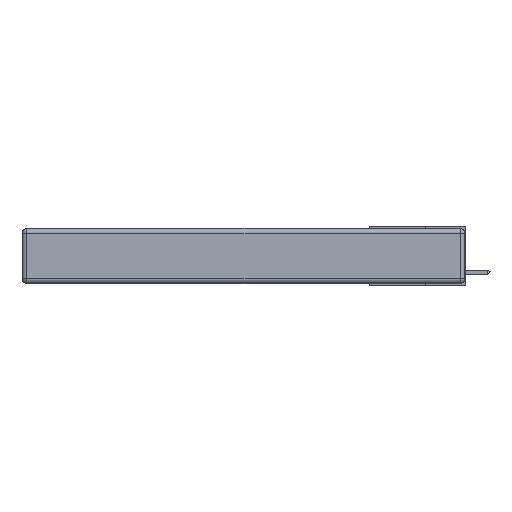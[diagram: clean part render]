
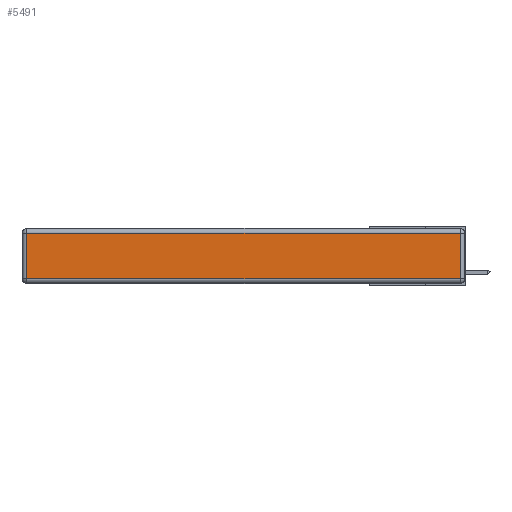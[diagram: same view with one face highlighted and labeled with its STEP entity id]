
A CAD part, left-side view. The second image highlights one B-rep face of the part: STEP entity #5491.
In plain terms, the highlighted planar face has unit normal (-1, 0, 0).
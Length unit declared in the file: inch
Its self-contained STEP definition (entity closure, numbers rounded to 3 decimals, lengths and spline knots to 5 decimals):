
#33 = DIRECTION ( 'NONE',  ( -1., 0., 0. ) ) ;
#1209 = VECTOR ( 'NONE', #25059, 39.37008 ) ;
#1692 = ORIENTED_EDGE ( 'NONE', *, *, #24910, .T. ) ;
#2163 = VERTEX_POINT ( 'NONE', #10046 ) ;
#3005 = ORIENTED_EDGE ( 'NONE', *, *, #19222, .T. ) ;
#4175 = CARTESIAN_POINT ( 'NONE',  ( 0., 0.03, -0.343 ) ) ;
#5222 = LINE ( 'NONE', #27090, #27977 ) ;
#5284 = CARTESIAN_POINT ( 'NONE',  ( 0., 2.72, -0.313 ) ) ;
#5491 = ADVANCED_FACE ( 'NONE', ( #24937 ), #19832, .T. ) ;
#6596 = LINE ( 'NONE', #17344, #19041 ) ;
#8658 = EDGE_CURVE ( 'NONE', #2163, #19083, #11894, .T. ) ;
#10046 = CARTESIAN_POINT ( 'NONE',  ( 0., 0.03, -0.313 ) ) ;
#10076 = AXIS2_PLACEMENT_3D ( 'NONE', #19945, #33, #22165 ) ;
#10414 = EDGE_CURVE ( 'NONE', #16299, #2163, #5222, .T. ) ;
#10538 = CARTESIAN_POINT ( 'NONE',  ( 0., 0.03, -0.03 ) ) ;
#10626 = DIRECTION ( 'NONE',  ( 0., 0., 1. ) ) ;
#11271 = EDGE_LOOP ( 'NONE', ( #21845, #22666, #1692, #3005 ) ) ;
#11894 = LINE ( 'NONE', #4175, #26020 ) ;
#12924 = LINE ( 'NONE', #22753, #1209 ) ;
#13142 = VERTEX_POINT ( 'NONE', #20031 ) ;
#16299 = VERTEX_POINT ( 'NONE', #5284 ) ;
#17059 = DIRECTION ( 'NONE',  ( 0., 0., -1. ) ) ;
#17344 = CARTESIAN_POINT ( 'NONE',  ( 0., 2.72, -0.343 ) ) ;
#19041 = VECTOR ( 'NONE', #17059, 39.37008 ) ;
#19083 = VERTEX_POINT ( 'NONE', #10538 ) ;
#19222 = EDGE_CURVE ( 'NONE', #13142, #16299, #6596, .T. ) ;
#19832 = PLANE ( 'NONE',  #10076 ) ;
#19945 = CARTESIAN_POINT ( 'NONE',  ( 0., 0., -0.343 ) ) ;
#20031 = CARTESIAN_POINT ( 'NONE',  ( 0., 2.72, -0.03 ) ) ;
#21845 = ORIENTED_EDGE ( 'NONE', *, *, #10414, .T. ) ;
#22165 = DIRECTION ( 'NONE',  ( 0., 0., 1. ) ) ;
#22666 = ORIENTED_EDGE ( 'NONE', *, *, #8658, .T. ) ;
#22753 = CARTESIAN_POINT ( 'NONE',  ( 0., 2.75, -0.03 ) ) ;
#24910 = EDGE_CURVE ( 'NONE', #19083, #13142, #12924, .T. ) ;
#24937 = FACE_OUTER_BOUND ( 'NONE', #11271, .T. ) ;
#25059 = DIRECTION ( 'NONE',  ( 0., 1., 0. ) ) ;
#26020 = VECTOR ( 'NONE', #10626, 39.37008 ) ;
#26823 = DIRECTION ( 'NONE',  ( 0., -1., 0. ) ) ;
#27090 = CARTESIAN_POINT ( 'NONE',  ( 0., 0., -0.313 ) ) ;
#27977 = VECTOR ( 'NONE', #26823, 39.37008 ) ;
